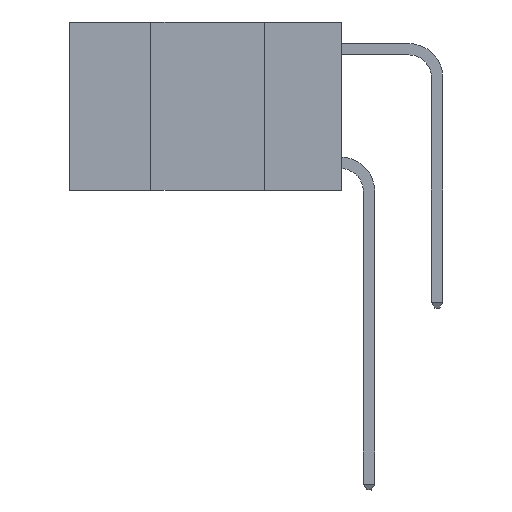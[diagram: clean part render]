
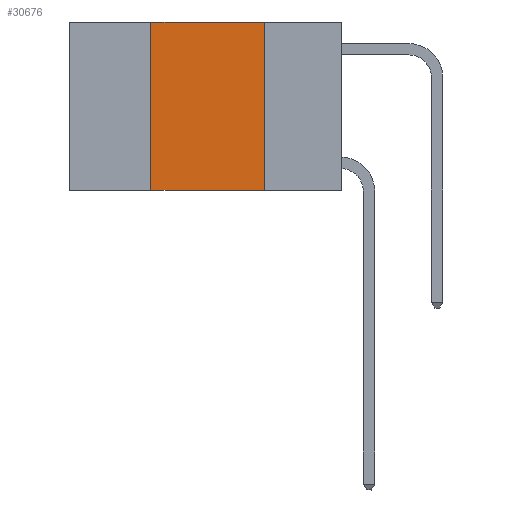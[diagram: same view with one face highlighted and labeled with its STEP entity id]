
A CAD part, left-side view. The second image highlights one B-rep face of the part: STEP entity #30676.
In plain terms, the highlighted planar face has unit normal (-1, 0, 0).
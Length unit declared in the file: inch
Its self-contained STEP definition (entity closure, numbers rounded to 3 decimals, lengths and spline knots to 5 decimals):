
#2600 = CARTESIAN_POINT ( 'NONE',  ( 0., 0.6, 0. ) ) ;
#3744 = VERTEX_POINT ( 'NONE', #24289 ) ;
#4258 = EDGE_CURVE ( 'NONE', #25418, #3744, #5960, .T. ) ;
#4406 = ORIENTED_EDGE ( 'NONE', *, *, #28595, .F. ) ;
#5588 = AXIS2_PLACEMENT_3D ( 'NONE', #22168, #22389, #9659 ) ;
#5941 = CARTESIAN_POINT ( 'NONE',  ( 0., 0.6, -0.37 ) ) ;
#5960 = LINE ( 'NONE', #5941, #11136 ) ;
#7289 = VECTOR ( 'NONE', #29204, 39.37008 ) ;
#7518 = EDGE_CURVE ( 'NONE', #8681, #22115, #21195, .T. ) ;
#7766 = VECTOR ( 'NONE', #22266, 39.37008 ) ;
#8681 = VERTEX_POINT ( 'NONE', #24584 ) ;
#9659 = DIRECTION ( 'NONE',  ( 0., 0., -1. ) ) ;
#11136 = VECTOR ( 'NONE', #27148, 39.37008 ) ;
#11168 = ORIENTED_EDGE ( 'NONE', *, *, #15624, .F. ) ;
#15360 = VECTOR ( 'NONE', #30839, 39.37008 ) ;
#15624 = EDGE_CURVE ( 'NONE', #25418, #8681, #23824, .T. ) ;
#16333 = CARTESIAN_POINT ( 'NONE',  ( 0., 0.17, 0. ) ) ;
#16346 = ORIENTED_EDGE ( 'NONE', *, *, #7518, .F. ) ;
#16550 = CARTESIAN_POINT ( 'NONE',  ( 0., 0.42, 0. ) ) ;
#21195 = LINE ( 'NONE', #2600, #7766 ) ;
#22115 = VERTEX_POINT ( 'NONE', #16333 ) ;
#22168 = CARTESIAN_POINT ( 'NONE',  ( 0., 0.6, 0. ) ) ;
#22266 = DIRECTION ( 'NONE',  ( 0., -1., 0. ) ) ;
#22389 = DIRECTION ( 'NONE',  ( 1., 0., 0. ) ) ;
#23824 = LINE ( 'NONE', #16550, #7289 ) ;
#23912 = FACE_OUTER_BOUND ( 'NONE', #29804, .T. ) ;
#24289 = CARTESIAN_POINT ( 'NONE',  ( 0., 0.17, -0.37 ) ) ;
#24584 = CARTESIAN_POINT ( 'NONE',  ( 0., 0.42, 0. ) ) ;
#25418 = VERTEX_POINT ( 'NONE', #31608 ) ;
#26909 = ORIENTED_EDGE ( 'NONE', *, *, #4258, .T. ) ;
#27148 = DIRECTION ( 'NONE',  ( 0., -1., 0. ) ) ;
#28595 = EDGE_CURVE ( 'NONE', #22115, #3744, #29555, .T. ) ;
#29204 = DIRECTION ( 'NONE',  ( 0., 0., 1. ) ) ;
#29555 = LINE ( 'NONE', #31164, #15360 ) ;
#29804 = EDGE_LOOP ( 'NONE', ( #4406, #16346, #11168, #26909 ) ) ;
#30125 = PLANE ( 'NONE',  #5588 ) ;
#30676 = ADVANCED_FACE ( 'NONE', ( #23912 ), #30125, .F. ) ;
#30839 = DIRECTION ( 'NONE',  ( 0., 0., -1. ) ) ;
#31164 = CARTESIAN_POINT ( 'NONE',  ( 0., 0.17, 0. ) ) ;
#31608 = CARTESIAN_POINT ( 'NONE',  ( 0., 0.42, -0.37 ) ) ;
